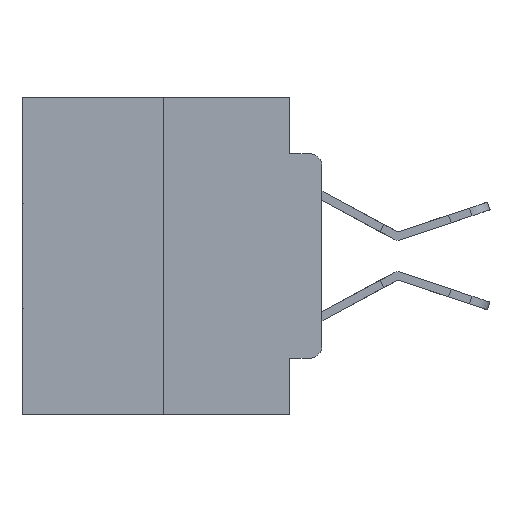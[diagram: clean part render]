
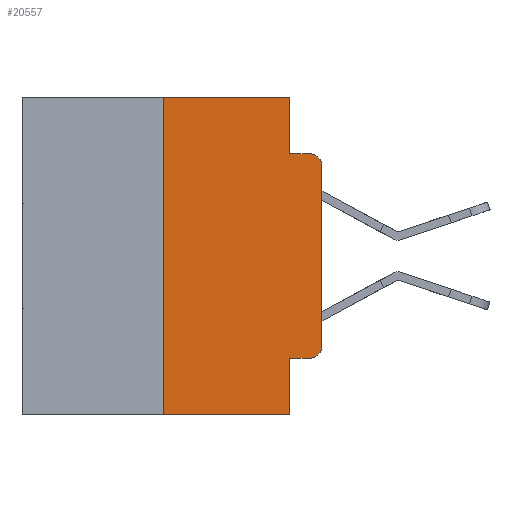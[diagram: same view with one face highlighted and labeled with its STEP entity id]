
A CAD part, left-side view. The second image highlights one B-rep face of the part: STEP entity #20557.
In plain terms, the highlighted planar face has unit normal (-1, 0, 0).
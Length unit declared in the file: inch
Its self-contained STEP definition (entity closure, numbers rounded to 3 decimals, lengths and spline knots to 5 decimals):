
#401 = VERTEX_POINT ( 'NONE', #3809 ) ;
#699 = EDGE_LOOP ( 'NONE', ( #2774, #25014, #16945, #9927, #9110, #11185, #11381, #7963, #20580, #25801 ) ) ;
#2196 = CARTESIAN_POINT ( 'NONE',  ( 0., 0.051, -0.0885 ) ) ;
#2774 = ORIENTED_EDGE ( 'NONE', *, *, #11991, .T. ) ;
#2895 = CARTESIAN_POINT ( 'NONE',  ( 0., 0.473, 0. ) ) ;
#3279 = AXIS2_PLACEMENT_3D ( 'NONE', #12956, #15263, #29120 ) ;
#3297 = CARTESIAN_POINT ( 'NONE',  ( 0., 0.473, -0.5 ) ) ;
#3381 = CARTESIAN_POINT ( 'NONE',  ( 0., 0.051, -0.4115 ) ) ;
#3809 = CARTESIAN_POINT ( 'NONE',  ( 0., 0.02, -0.0885 ) ) ;
#4861 = CARTESIAN_POINT ( 'NONE',  ( 0., 0.051, 0. ) ) ;
#4975 = CARTESIAN_POINT ( 'NONE',  ( 0., 0.051, 0. ) ) ;
#5964 = VERTEX_POINT ( 'NONE', #27125 ) ;
#6048 = CARTESIAN_POINT ( 'NONE',  ( 0., 0.25, -0.5 ) ) ;
#6324 = VECTOR ( 'NONE', #27103, 39.37008 ) ;
#6480 = EDGE_CURVE ( 'NONE', #11490, #19959, #10504, .T. ) ;
#7377 = LINE ( 'NONE', #24785, #6324 ) ;
#7461 = CIRCLE ( 'NONE', #29836, 0.02 ) ;
#7963 = ORIENTED_EDGE ( 'NONE', *, *, #8945, .F. ) ;
#8317 = CARTESIAN_POINT ( 'NONE',  ( 0., 0.473, 0. ) ) ;
#8693 = EDGE_CURVE ( 'NONE', #24365, #401, #7461, .T. ) ;
#8945 = EDGE_CURVE ( 'NONE', #27214, #23110, #22988, .T. ) ;
#9110 = ORIENTED_EDGE ( 'NONE', *, *, #13991, .F. ) ;
#9237 = DIRECTION ( 'NONE',  ( -1., 0., 0. ) ) ;
#9462 = VECTOR ( 'NONE', #20950, 39.37008 ) ;
#9466 = AXIS2_PLACEMENT_3D ( 'NONE', #2895, #9709, #25863 ) ;
#9709 = DIRECTION ( 'NONE',  ( 1., 0., 0. ) ) ;
#9726 = EDGE_CURVE ( 'NONE', #28378, #401, #27650, .T. ) ;
#9874 = LINE ( 'NONE', #8317, #15312 ) ;
#9927 = ORIENTED_EDGE ( 'NONE', *, *, #26404, .F. ) ;
#10197 = LINE ( 'NONE', #4861, #9462 ) ;
#10504 = LINE ( 'NONE', #14890, #26003 ) ;
#10848 = DIRECTION ( 'NONE',  ( 0., -1., 0. ) ) ;
#10926 = EDGE_CURVE ( 'NONE', #27214, #22685, #7377, .T. ) ;
#11185 = ORIENTED_EDGE ( 'NONE', *, *, #6480, .F. ) ;
#11381 = ORIENTED_EDGE ( 'NONE', *, *, #12714, .T. ) ;
#11490 = VERTEX_POINT ( 'NONE', #6048 ) ;
#11991 = EDGE_CURVE ( 'NONE', #15230, #24365, #20840, .T. ) ;
#12449 = FACE_OUTER_BOUND ( 'NONE', #699, .T. ) ;
#12714 = EDGE_CURVE ( 'NONE', #11490, #23110, #22609, .T. ) ;
#12956 = CARTESIAN_POINT ( 'NONE',  ( 0., 0.02, -0.3915 ) ) ;
#13110 = CARTESIAN_POINT ( 'NONE',  ( 0., 0.02, -0.1085 ) ) ;
#13991 = EDGE_CURVE ( 'NONE', #19959, #5964, #9874, .T. ) ;
#14303 = VECTOR ( 'NONE', #21983, 39.37008 ) ;
#14404 = CARTESIAN_POINT ( 'NONE',  ( 0., 0.25, 0. ) ) ;
#14543 = CARTESIAN_POINT ( 'NONE',  ( 0., 0., 0. ) ) ;
#14662 = DIRECTION ( 'NONE',  ( 0., -1., 0. ) ) ;
#14890 = CARTESIAN_POINT ( 'NONE',  ( 0., 0.25, 0. ) ) ;
#14988 = DIRECTION ( 'NONE',  ( 0., 0., 1. ) ) ;
#15216 = CARTESIAN_POINT ( 'NONE',  ( 0., 0.051, -0.0885 ) ) ;
#15230 = VERTEX_POINT ( 'NONE', #21103 ) ;
#15263 = DIRECTION ( 'NONE',  ( -1., 0., 0. ) ) ;
#15312 = VECTOR ( 'NONE', #10848, 39.37008 ) ;
#16857 = VECTOR ( 'NONE', #23466, 39.37008 ) ;
#16945 = ORIENTED_EDGE ( 'NONE', *, *, #9726, .F. ) ;
#17218 = VECTOR ( 'NONE', #14662, 39.37008 ) ;
#17476 = CARTESIAN_POINT ( 'NONE',  ( 0., 0.051, -0.5 ) ) ;
#17607 = CARTESIAN_POINT ( 'NONE',  ( 0., 0.02, -0.4115 ) ) ;
#18152 = DIRECTION ( 'NONE',  ( 0., 0., -1. ) ) ;
#18348 = CIRCLE ( 'NONE', #3279, 0.02 ) ;
#19058 = VECTOR ( 'NONE', #21705, 39.37008 ) ;
#19959 = VERTEX_POINT ( 'NONE', #14404 ) ;
#20557 = ADVANCED_FACE ( 'NONE', ( #12449 ), #21132, .F. ) ;
#20580 = ORIENTED_EDGE ( 'NONE', *, *, #10926, .T. ) ;
#20840 = LINE ( 'NONE', #14543, #19058 ) ;
#20950 = DIRECTION ( 'NONE',  ( 0., 0., -1. ) ) ;
#21103 = CARTESIAN_POINT ( 'NONE',  ( 0., 0., -0.3915 ) ) ;
#21132 = PLANE ( 'NONE',  #9466 ) ;
#21705 = DIRECTION ( 'NONE',  ( 0., 0., 1. ) ) ;
#21983 = DIRECTION ( 'NONE',  ( 0., -1., 0. ) ) ;
#22609 = LINE ( 'NONE', #3297, #17218 ) ;
#22685 = VERTEX_POINT ( 'NONE', #17607 ) ;
#22988 = LINE ( 'NONE', #4975, #16857 ) ;
#23110 = VERTEX_POINT ( 'NONE', #17476 ) ;
#23466 = DIRECTION ( 'NONE',  ( 0., 0., -1. ) ) ;
#24365 = VERTEX_POINT ( 'NONE', #28760 ) ;
#24785 = CARTESIAN_POINT ( 'NONE',  ( 0., 0.051, -0.4115 ) ) ;
#25014 = ORIENTED_EDGE ( 'NONE', *, *, #8693, .T. ) ;
#25801 = ORIENTED_EDGE ( 'NONE', *, *, #28887, .T. ) ;
#25863 = DIRECTION ( 'NONE',  ( 0., 0., -1. ) ) ;
#26003 = VECTOR ( 'NONE', #14988, 39.37008 ) ;
#26404 = EDGE_CURVE ( 'NONE', #5964, #28378, #10197, .T. ) ;
#27103 = DIRECTION ( 'NONE',  ( 0., -1., 0. ) ) ;
#27125 = CARTESIAN_POINT ( 'NONE',  ( 0., 0.051, 0. ) ) ;
#27214 = VERTEX_POINT ( 'NONE', #3381 ) ;
#27650 = LINE ( 'NONE', #15216, #14303 ) ;
#28378 = VERTEX_POINT ( 'NONE', #2196 ) ;
#28760 = CARTESIAN_POINT ( 'NONE',  ( 0., 0., -0.1085 ) ) ;
#28887 = EDGE_CURVE ( 'NONE', #22685, #15230, #18348, .T. ) ;
#29120 = DIRECTION ( 'NONE',  ( 0., 0., -1. ) ) ;
#29836 = AXIS2_PLACEMENT_3D ( 'NONE', #13110, #9237, #18152 ) ;
